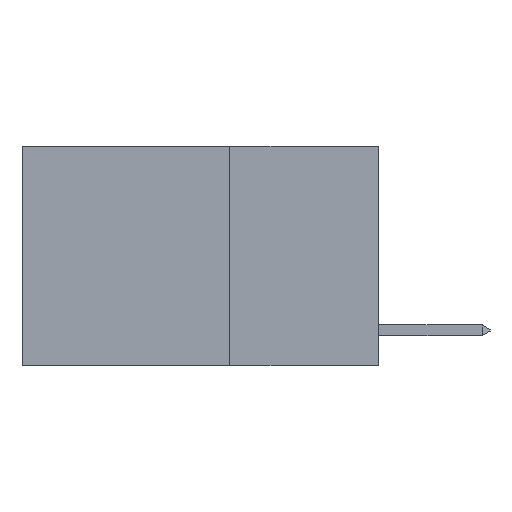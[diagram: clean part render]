
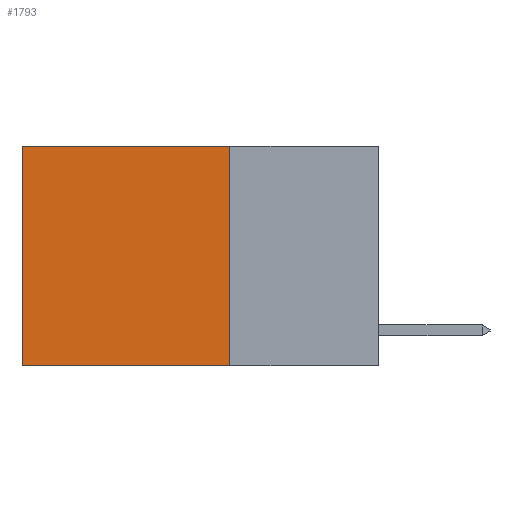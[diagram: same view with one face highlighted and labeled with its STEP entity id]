
A CAD part, left-side view. The second image highlights one B-rep face of the part: STEP entity #1793.
In plain terms, the highlighted planar face has unit normal (-1, 0, 0).
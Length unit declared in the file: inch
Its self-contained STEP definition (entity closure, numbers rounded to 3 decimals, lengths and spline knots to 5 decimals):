
#392 = LINE ( 'NONE', #6521, #8684 ) ;
#1059 = PLANE ( 'NONE',  #1552 ) ;
#1516 = VECTOR ( 'NONE', #9901, 39.37008 ) ;
#1552 = AXIS2_PLACEMENT_3D ( 'NONE', #5104, #1909, #7458 ) ;
#1688 = LINE ( 'NONE', #9703, #7525 ) ;
#1793 = ADVANCED_FACE ( 'NONE', ( #3873 ), #1059, .F. ) ;
#1909 = DIRECTION ( 'NONE',  ( 1., 0., 0. ) ) ;
#2080 = CARTESIAN_POINT ( 'NONE',  ( 0.2625, 0.6, 0. ) ) ;
#2341 = VECTOR ( 'NONE', #4830, 39.37008 ) ;
#2347 = EDGE_CURVE ( 'NONE', #3513, #2605, #392, .T. ) ;
#2605 = VERTEX_POINT ( 'NONE', #2080 ) ;
#2647 = CARTESIAN_POINT ( 'NONE',  ( 0.2625, 0.25, -0.37 ) ) ;
#3278 = ORIENTED_EDGE ( 'NONE', *, *, #5358, .F. ) ;
#3513 = VERTEX_POINT ( 'NONE', #4187 ) ;
#3514 = VERTEX_POINT ( 'NONE', #2647 ) ;
#3873 = FACE_OUTER_BOUND ( 'NONE', #5973, .T. ) ;
#4001 = EDGE_CURVE ( 'NONE', #2605, #5764, #6298, .T. ) ;
#4154 = ORIENTED_EDGE ( 'NONE', *, *, #2347, .T. ) ;
#4187 = CARTESIAN_POINT ( 'NONE',  ( 0.2625, 0.25, 0. ) ) ;
#4204 = DIRECTION ( 'NONE',  ( 0., 1., 0. ) ) ;
#4830 = DIRECTION ( 'NONE',  ( 0., 0., -1. ) ) ;
#4935 = CARTESIAN_POINT ( 'NONE',  ( 0.2625, 0.6, -0.37 ) ) ;
#5104 = CARTESIAN_POINT ( 'NONE',  ( 0.2625, 0.25, 0. ) ) ;
#5358 = EDGE_CURVE ( 'NONE', #3513, #3514, #9468, .T. ) ;
#5653 = ORIENTED_EDGE ( 'NONE', *, *, #4001, .T. ) ;
#5764 = VERTEX_POINT ( 'NONE', #4935 ) ;
#5973 = EDGE_LOOP ( 'NONE', ( #5653, #10202, #3278, #4154 ) ) ;
#6298 = LINE ( 'NONE', #7167, #2341 ) ;
#6521 = CARTESIAN_POINT ( 'NONE',  ( 0.2625, 0.25, 0. ) ) ;
#7167 = CARTESIAN_POINT ( 'NONE',  ( 0.2625, 0.6, 0. ) ) ;
#7458 = DIRECTION ( 'NONE',  ( 0., 0., -1. ) ) ;
#7525 = VECTOR ( 'NONE', #4204, 39.37008 ) ;
#8121 = DIRECTION ( 'NONE',  ( 0., 1., 0. ) ) ;
#8684 = VECTOR ( 'NONE', #8121, 39.37008 ) ;
#8992 = EDGE_CURVE ( 'NONE', #3514, #5764, #1688, .T. ) ;
#9114 = CARTESIAN_POINT ( 'NONE',  ( 0.2625, 0.25, 0. ) ) ;
#9468 = LINE ( 'NONE', #9114, #1516 ) ;
#9703 = CARTESIAN_POINT ( 'NONE',  ( 0.2625, 0.25, -0.37 ) ) ;
#9901 = DIRECTION ( 'NONE',  ( 0., 0., -1. ) ) ;
#10202 = ORIENTED_EDGE ( 'NONE', *, *, #8992, .F. ) ;
